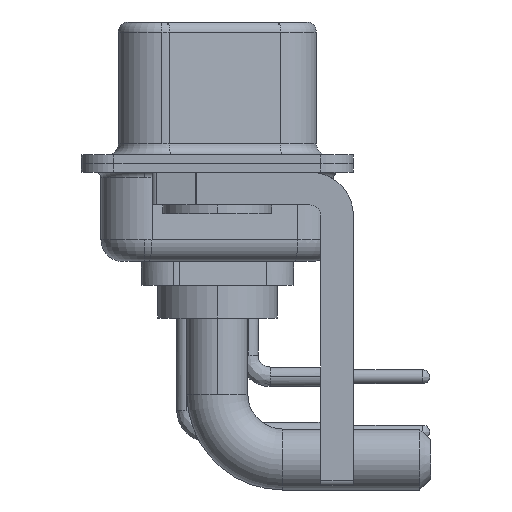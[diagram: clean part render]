
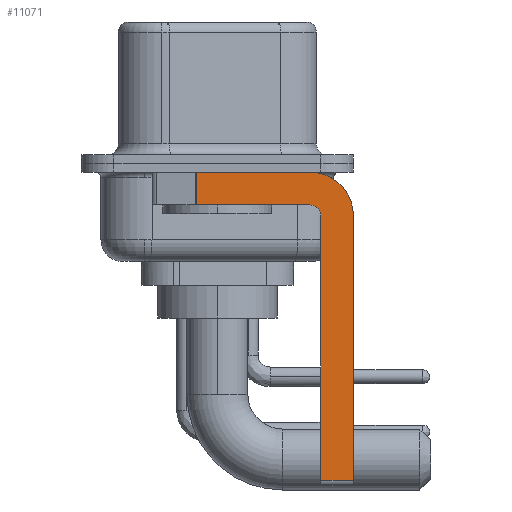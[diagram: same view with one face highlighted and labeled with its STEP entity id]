
A CAD part, left-side view. The second image highlights one B-rep face of the part: STEP entity #11071.
In plain terms, the highlighted planar face has unit normal (-1, 0, 0).
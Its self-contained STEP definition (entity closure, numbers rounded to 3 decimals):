
#1010 = LINE ( 'NONE', #13796, #23262 ) ;
#1258 = FACE_OUTER_BOUND ( 'NONE', #1676, .T. ) ;
#1547 = LINE ( 'NONE', #8086, #15793 ) ;
#1647 = LINE ( 'NONE', #19200, #2188 ) ;
#1676 = EDGE_LOOP ( 'NONE', ( #18689, #5465, #8486, #12434, #14626, #11837, #13814, #6309 ) ) ;
#1839 = CARTESIAN_POINT ( 'NONE',  ( -2.9, -4.25, -0.4 ) ) ;
#2104 = VERTEX_POINT ( 'NONE', #1839 ) ;
#2188 = VECTOR ( 'NONE', #10495, 1000. ) ;
#2928 = CARTESIAN_POINT ( 'NONE',  ( -2.9, 0.978, -1.9 ) ) ;
#2969 = CARTESIAN_POINT ( 'NONE',  ( -2.9, -4.25, -14.55 ) ) ;
#3169 = EDGE_CURVE ( 'NONE', #20145, #26670, #1647, .T. ) ;
#3250 = DIRECTION ( 'NONE',  ( 0., 0., -1. ) ) ;
#3393 = DIRECTION ( 'NONE',  ( 1., 0., 0. ) ) ;
#3724 = CARTESIAN_POINT ( 'NONE',  ( -2.9, -4.75, -14.55 ) ) ;
#3901 = EDGE_CURVE ( 'NONE', #18499, #14970, #15363, .T. ) ;
#4208 = VERTEX_POINT ( 'NONE', #7558 ) ;
#5397 = AXIS2_PLACEMENT_3D ( 'NONE', #27198, #3393, #3250 ) ;
#5465 = ORIENTED_EDGE ( 'NONE', *, *, #7022, .T. ) ;
#6309 = ORIENTED_EDGE ( 'NONE', *, *, #27291, .F. ) ;
#6470 = DIRECTION ( 'NONE',  ( 0., 0., 1. ) ) ;
#6967 = CARTESIAN_POINT ( 'NONE',  ( -2.9, -4.25, -2.4 ) ) ;
#7022 = EDGE_CURVE ( 'NONE', #21690, #14970, #1010, .T. ) ;
#7111 = DIRECTION ( 'NONE',  ( 0., 0., -1. ) ) ;
#7243 = LINE ( 'NONE', #24777, #12002 ) ;
#7558 = CARTESIAN_POINT ( 'NONE',  ( -2.9, -4.75, -2.4 ) ) ;
#8086 = CARTESIAN_POINT ( 'NONE',  ( -2.9, -4.75, -14.8 ) ) ;
#8486 = ORIENTED_EDGE ( 'NONE', *, *, #3901, .F. ) ;
#8869 = VERTEX_POINT ( 'NONE', #3724 ) ;
#9042 = VECTOR ( 'NONE', #9504, 1000. ) ;
#9504 = DIRECTION ( 'NONE',  ( 0., -1., 0. ) ) ;
#10495 = DIRECTION ( 'NONE',  ( 0., 0., -1. ) ) ;
#10663 = CIRCLE ( 'NONE', #24551, 0.5 ) ;
#11071 = ADVANCED_FACE ( 'NONE', ( #1258 ), #15801, .F. ) ;
#11837 = ORIENTED_EDGE ( 'NONE', *, *, #26273, .T. ) ;
#11878 = DIRECTION ( 'NONE',  ( 0., -1., 0. ) ) ;
#12002 = VECTOR ( 'NONE', #11878, 1000. ) ;
#12434 = ORIENTED_EDGE ( 'NONE', *, *, #20930, .F. ) ;
#12731 = DIRECTION ( 'NONE',  ( 0., 0., 1. ) ) ;
#13796 = CARTESIAN_POINT ( 'NONE',  ( -2.9, 0.978, -1.9 ) ) ;
#13814 = ORIENTED_EDGE ( 'NONE', *, *, #3169, .F. ) ;
#14145 = LINE ( 'NONE', #2969, #9042 ) ;
#14626 = ORIENTED_EDGE ( 'NONE', *, *, #22070, .F. ) ;
#14970 = VERTEX_POINT ( 'NONE', #2928 ) ;
#15363 = LINE ( 'NONE', #24213, #21221 ) ;
#15793 = VECTOR ( 'NONE', #12731, 1000. ) ;
#15801 = PLANE ( 'NONE',  #17852 ) ;
#17631 = CARTESIAN_POINT ( 'NONE',  ( -2.9, -4.25, -2.4 ) ) ;
#17688 = DIRECTION ( 'NONE',  ( 0., 1., 0. ) ) ;
#17852 = AXIS2_PLACEMENT_3D ( 'NONE', #6967, #23162, #7111 ) ;
#18499 = VERTEX_POINT ( 'NONE', #28081 ) ;
#18689 = ORIENTED_EDGE ( 'NONE', *, *, #19767, .F. ) ;
#19200 = CARTESIAN_POINT ( 'NONE',  ( -2.9, -6.25, -2.4 ) ) ;
#19767 = EDGE_CURVE ( 'NONE', #21690, #2104, #7243, .T. ) ;
#20145 = VERTEX_POINT ( 'NONE', #25551 ) ;
#20930 = EDGE_CURVE ( 'NONE', #4208, #18499, #10663, .T. ) ;
#21221 = VECTOR ( 'NONE', #17688, 1000. ) ;
#21690 = VERTEX_POINT ( 'NONE', #26076 ) ;
#21715 = CARTESIAN_POINT ( 'NONE',  ( -2.9, -6.25, -14.55 ) ) ;
#22070 = EDGE_CURVE ( 'NONE', #8869, #4208, #1547, .T. ) ;
#22148 = DIRECTION ( 'NONE',  ( -1., 0., 0. ) ) ;
#23162 = DIRECTION ( 'NONE',  ( 1., 0., 0. ) ) ;
#23262 = VECTOR ( 'NONE', #25086, 1000. ) ;
#24213 = CARTESIAN_POINT ( 'NONE',  ( -2.9, -4.25, -1.9 ) ) ;
#24551 = AXIS2_PLACEMENT_3D ( 'NONE', #17631, #22148, #6470 ) ;
#24777 = CARTESIAN_POINT ( 'NONE',  ( -2.9, 3., -0.4 ) ) ;
#25086 = DIRECTION ( 'NONE',  ( 0., 0., -1. ) ) ;
#25551 = CARTESIAN_POINT ( 'NONE',  ( -2.9, -6.25, -2.4 ) ) ;
#26076 = CARTESIAN_POINT ( 'NONE',  ( -2.9, 0.978, -0.4 ) ) ;
#26273 = EDGE_CURVE ( 'NONE', #8869, #26670, #14145, .T. ) ;
#26670 = VERTEX_POINT ( 'NONE', #21715 ) ;
#27198 = CARTESIAN_POINT ( 'NONE',  ( -2.9, -4.25, -2.4 ) ) ;
#27291 = EDGE_CURVE ( 'NONE', #2104, #20145, #28116, .T. ) ;
#28081 = CARTESIAN_POINT ( 'NONE',  ( -2.9, -4.25, -1.9 ) ) ;
#28116 = CIRCLE ( 'NONE', #5397, 2. ) ;
